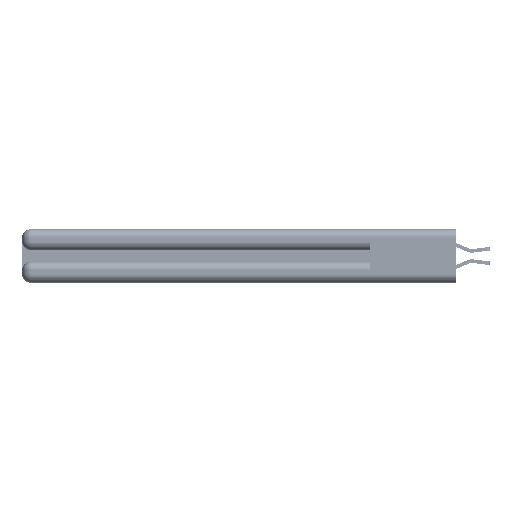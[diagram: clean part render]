
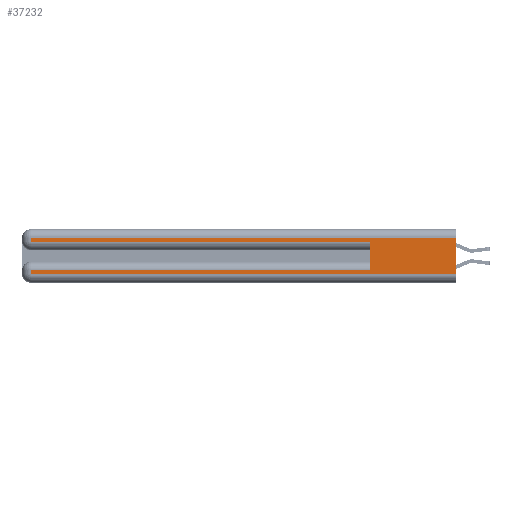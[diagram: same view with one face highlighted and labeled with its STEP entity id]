
A CAD part, left-side view. The second image highlights one B-rep face of the part: STEP entity #37232.
In plain terms, the highlighted planar face has unit normal (-1, 0, 0).
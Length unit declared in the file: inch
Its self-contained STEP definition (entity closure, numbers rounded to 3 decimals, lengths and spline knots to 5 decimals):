
#107 = EDGE_CURVE ( 'NONE', #25764, #49707, #37300, .T. ) ;
#247 = CARTESIAN_POINT ( 'NONE',  ( 0., 2.94, 0.06 ) ) ;
#378 = CARTESIAN_POINT ( 'NONE',  ( 0., 0., 0.285 ) ) ;
#564 = PLANE ( 'NONE',  #25155 ) ;
#3069 = LINE ( 'NONE', #13043, #11854 ) ;
#3438 = VERTEX_POINT ( 'NONE', #11687 ) ;
#3534 = DIRECTION ( 'NONE',  ( 0., 1., 0. ) ) ;
#5896 = ORIENTED_EDGE ( 'NONE', *, *, #14298, .F. ) ;
#6669 = EDGE_CURVE ( 'NONE', #20298, #25764, #3069, .T. ) ;
#6754 = FACE_OUTER_BOUND ( 'NONE', #32112, .T. ) ;
#7541 = LINE ( 'NONE', #54733, #29016 ) ;
#7702 = ORIENTED_EDGE ( 'NONE', *, *, #107, .T. ) ;
#8671 = DIRECTION ( 'NONE',  ( 0., 0., -1. ) ) ;
#9241 = DIRECTION ( 'NONE',  ( 1., 0., 0. ) ) ;
#11687 = CARTESIAN_POINT ( 'NONE',  ( 0., 0., 0.31 ) ) ;
#11854 = VECTOR ( 'NONE', #8671, 39.37008 ) ;
#13043 = CARTESIAN_POINT ( 'NONE',  ( 0., 2.94, 0.37 ) ) ;
#13292 = ORIENTED_EDGE ( 'NONE', *, *, #47507, .T. ) ;
#13350 = ORIENTED_EDGE ( 'NONE', *, *, #37212, .T. ) ;
#14298 = EDGE_CURVE ( 'NONE', #27641, #23830, #38192, .T. ) ;
#14569 = VECTOR ( 'NONE', #15962, 39.37008 ) ;
#15962 = DIRECTION ( 'NONE',  ( 0., -1., 0. ) ) ;
#16742 = ORIENTED_EDGE ( 'NONE', *, *, #19420, .T. ) ;
#18028 = CARTESIAN_POINT ( 'NONE',  ( 0., 0.6, 0.285 ) ) ;
#18382 = LINE ( 'NONE', #48518, #50950 ) ;
#19420 = EDGE_CURVE ( 'NONE', #34061, #27108, #18382, .T. ) ;
#20298 = VERTEX_POINT ( 'NONE', #46213 ) ;
#22072 = DIRECTION ( 'NONE',  ( 0., -1., 0. ) ) ;
#23830 = VERTEX_POINT ( 'NONE', #18028 ) ;
#24755 = CARTESIAN_POINT ( 'NONE',  ( 0., 0.6, 0.085 ) ) ;
#25155 = AXIS2_PLACEMENT_3D ( 'NONE', #30626, #9241, #39184 ) ;
#25764 = VERTEX_POINT ( 'NONE', #247 ) ;
#26840 = VECTOR ( 'NONE', #51213, 39.37008 ) ;
#27089 = VECTOR ( 'NONE', #29143, 39.37008 ) ;
#27108 = VERTEX_POINT ( 'NONE', #29639 ) ;
#27641 = VERTEX_POINT ( 'NONE', #24755 ) ;
#29016 = VECTOR ( 'NONE', #3534, 39.37008 ) ;
#29143 = DIRECTION ( 'NONE',  ( 0., 1., 0. ) ) ;
#29162 = EDGE_CURVE ( 'NONE', #3438, #49707, #46627, .T. ) ;
#29639 = CARTESIAN_POINT ( 'NONE',  ( 0., 2.94, 0.285 ) ) ;
#30626 = CARTESIAN_POINT ( 'NONE',  ( 0., 0., 0.37 ) ) ;
#31323 = CARTESIAN_POINT ( 'NONE',  ( 0., 0., 0.37 ) ) ;
#32112 = EDGE_LOOP ( 'NONE', ( #38648, #13292, #16742, #13350, #5896, #44062, #53830, #7702 ) ) ;
#34012 = VECTOR ( 'NONE', #35429, 39.37008 ) ;
#34061 = VERTEX_POINT ( 'NONE', #53271 ) ;
#35429 = DIRECTION ( 'NONE',  ( 0., 0., -1. ) ) ;
#37212 = EDGE_CURVE ( 'NONE', #27108, #23830, #52170, .T. ) ;
#37232 = ADVANCED_FACE ( 'NONE', ( #6754 ), #564, .F. ) ;
#37300 = LINE ( 'NONE', #50004, #14569 ) ;
#38192 = LINE ( 'NONE', #38444, #26840 ) ;
#38427 = LINE ( 'NONE', #46051, #27089 ) ;
#38444 = CARTESIAN_POINT ( 'NONE',  ( 0., 0.6, 0.145 ) ) ;
#38648 = ORIENTED_EDGE ( 'NONE', *, *, #29162, .F. ) ;
#39184 = DIRECTION ( 'NONE',  ( 0., 0., -1. ) ) ;
#43723 = CARTESIAN_POINT ( 'NONE',  ( 0., 0., 0.06 ) ) ;
#44062 = ORIENTED_EDGE ( 'NONE', *, *, #46845, .T. ) ;
#46051 = CARTESIAN_POINT ( 'NONE',  ( 0., 0., 0.085 ) ) ;
#46213 = CARTESIAN_POINT ( 'NONE',  ( 0., 2.94, 0.085 ) ) ;
#46627 = LINE ( 'NONE', #31323, #34012 ) ;
#46845 = EDGE_CURVE ( 'NONE', #27641, #20298, #38427, .T. ) ;
#47507 = EDGE_CURVE ( 'NONE', #3438, #34061, #7541, .T. ) ;
#48518 = CARTESIAN_POINT ( 'NONE',  ( 0., 2.94, 0.37 ) ) ;
#49707 = VERTEX_POINT ( 'NONE', #43723 ) ;
#50004 = CARTESIAN_POINT ( 'NONE',  ( 0., 0., 0.06 ) ) ;
#50842 = VECTOR ( 'NONE', #22072, 39.37008 ) ;
#50950 = VECTOR ( 'NONE', #52766, 39.37008 ) ;
#51213 = DIRECTION ( 'NONE',  ( 0., 0., 1. ) ) ;
#52170 = LINE ( 'NONE', #378, #50842 ) ;
#52766 = DIRECTION ( 'NONE',  ( 0., 0., -1. ) ) ;
#53271 = CARTESIAN_POINT ( 'NONE',  ( 0., 2.94, 0.31 ) ) ;
#53830 = ORIENTED_EDGE ( 'NONE', *, *, #6669, .T. ) ;
#54733 = CARTESIAN_POINT ( 'NONE',  ( 0., 0., 0.31 ) ) ;
